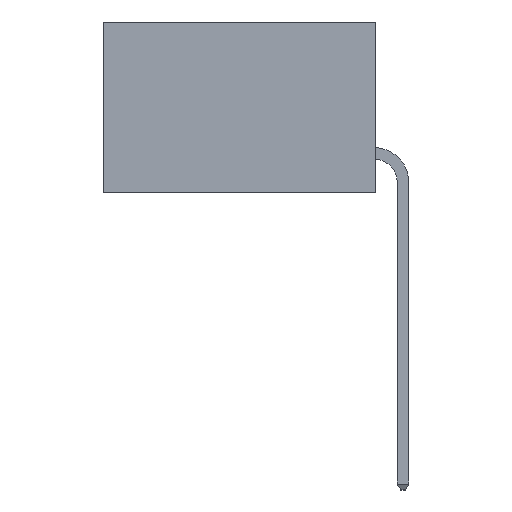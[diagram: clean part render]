
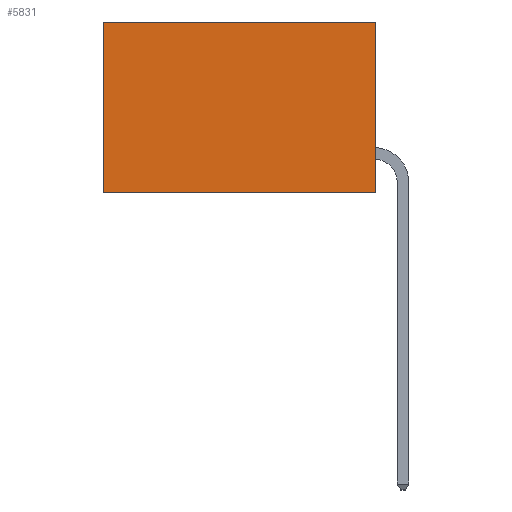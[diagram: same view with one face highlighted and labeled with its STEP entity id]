
A CAD part, left-side view. The second image highlights one B-rep face of the part: STEP entity #5831.
In plain terms, the highlighted planar face has unit normal (-1, 0, 0).
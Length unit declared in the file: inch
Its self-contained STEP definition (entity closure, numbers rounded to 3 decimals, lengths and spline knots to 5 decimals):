
#1575 = VECTOR ( 'NONE', #11018, 39.37008 ) ;
#1981 = FACE_OUTER_BOUND ( 'NONE', #10788, .T. ) ;
#2079 = CARTESIAN_POINT ( 'NONE',  ( 0.277, 0., 0. ) ) ;
#2480 = CARTESIAN_POINT ( 'NONE',  ( 0.277, 0., 0. ) ) ;
#2692 = LINE ( 'NONE', #12902, #16189 ) ;
#3009 = EDGE_CURVE ( 'NONE', #16238, #12510, #12198, .T. ) ;
#3380 = ORIENTED_EDGE ( 'NONE', *, *, #7265, .T. ) ;
#3471 = CARTESIAN_POINT ( 'NONE',  ( 0.277, 0., -0.37 ) ) ;
#3694 = LINE ( 'NONE', #3830, #17060 ) ;
#3772 = DIRECTION ( 'NONE',  ( 0., 0., -1. ) ) ;
#3830 = CARTESIAN_POINT ( 'NONE',  ( 0.277, 0.59, -0.37 ) ) ;
#4881 = CARTESIAN_POINT ( 'NONE',  ( 0.277, 0.59, 0. ) ) ;
#5099 = ORIENTED_EDGE ( 'NONE', *, *, #3009, .T. ) ;
#5282 = CARTESIAN_POINT ( 'NONE',  ( 0.277, 0., -0.37 ) ) ;
#5831 = ADVANCED_FACE ( 'NONE', ( #1981 ), #16626, .F. ) ;
#6602 = DIRECTION ( 'NONE',  ( 0., 0., -1. ) ) ;
#7265 = EDGE_CURVE ( 'NONE', #12510, #13191, #3694, .T. ) ;
#7753 = ORIENTED_EDGE ( 'NONE', *, *, #16478, .F. ) ;
#8678 = LINE ( 'NONE', #5282, #11353 ) ;
#10788 = EDGE_LOOP ( 'NONE', ( #3380, #12896, #7753, #5099 ) ) ;
#11003 = VERTEX_POINT ( 'NONE', #3471 ) ;
#11018 = DIRECTION ( 'NONE',  ( 0., 1., 0. ) ) ;
#11151 = EDGE_CURVE ( 'NONE', #11003, #13191, #2692, .T. ) ;
#11353 = VECTOR ( 'NONE', #6602, 39.37008 ) ;
#12198 = LINE ( 'NONE', #2480, #1575 ) ;
#12510 = VERTEX_POINT ( 'NONE', #4881 ) ;
#12602 = AXIS2_PLACEMENT_3D ( 'NONE', #16344, #15923, #15823 ) ;
#12896 = ORIENTED_EDGE ( 'NONE', *, *, #11151, .F. ) ;
#12902 = CARTESIAN_POINT ( 'NONE',  ( 0.277, 0., -0.37 ) ) ;
#13191 = VERTEX_POINT ( 'NONE', #16494 ) ;
#15823 = DIRECTION ( 'NONE',  ( 0., 0., -1. ) ) ;
#15923 = DIRECTION ( 'NONE',  ( 1., 0., 0. ) ) ;
#16189 = VECTOR ( 'NONE', #16747, 39.37008 ) ;
#16238 = VERTEX_POINT ( 'NONE', #2079 ) ;
#16344 = CARTESIAN_POINT ( 'NONE',  ( 0.277, 0., -0.37 ) ) ;
#16478 = EDGE_CURVE ( 'NONE', #16238, #11003, #8678, .T. ) ;
#16494 = CARTESIAN_POINT ( 'NONE',  ( 0.277, 0.59, -0.37 ) ) ;
#16626 = PLANE ( 'NONE',  #12602 ) ;
#16747 = DIRECTION ( 'NONE',  ( 0., 1., 0. ) ) ;
#17060 = VECTOR ( 'NONE', #3772, 39.37008 ) ;
